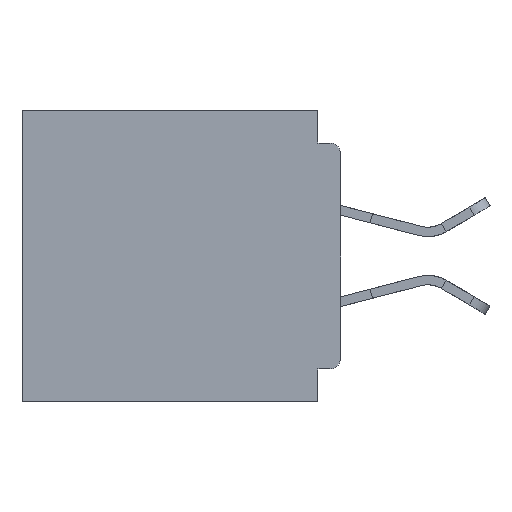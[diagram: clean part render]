
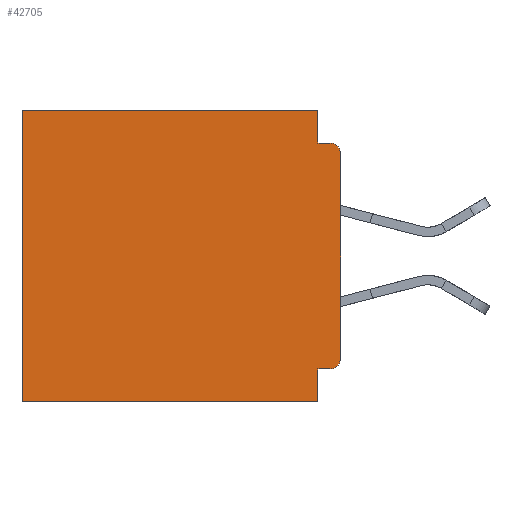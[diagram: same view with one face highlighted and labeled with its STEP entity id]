
A CAD part, left-side view. The second image highlights one B-rep face of the part: STEP entity #42705.
In plain terms, the highlighted planar face has unit normal (-1, 0, 0).
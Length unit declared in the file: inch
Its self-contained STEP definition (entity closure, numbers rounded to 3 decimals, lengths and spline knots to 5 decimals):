
#478 = ORIENTED_EDGE ( 'NONE', *, *, #38318, .T. ) ;
#631 = ORIENTED_EDGE ( 'NONE', *, *, #8554, .F. ) ;
#652 = ORIENTED_EDGE ( 'NONE', *, *, #33060, .F. ) ;
#1007 = ORIENTED_EDGE ( 'NONE', *, *, #11516, .F. ) ;
#1162 = DIRECTION ( 'NONE',  ( -1., 0., 0. ) ) ;
#1237 = DIRECTION ( 'NONE',  ( 0., 0., -1. ) ) ;
#1367 = LINE ( 'NONE', #6785, #37775 ) ;
#2070 = VERTEX_POINT ( 'NONE', #13846 ) ;
#2104 = LINE ( 'NONE', #34394, #11601 ) ;
#2105 = CARTESIAN_POINT ( 'NONE',  ( 0.3, 0.015, -0.045 ) ) ;
#2699 = VECTOR ( 'NONE', #28608, 39.37008 ) ;
#3477 = DIRECTION ( 'NONE',  ( 0., 0., -1. ) ) ;
#3554 = EDGE_CURVE ( 'NONE', #36889, #11849, #17380, .T. ) ;
#5534 = CARTESIAN_POINT ( 'NONE',  ( 0.3, 0., -0.4 ) ) ;
#6660 = VECTOR ( 'NONE', #39659, 39.37008 ) ;
#6785 = CARTESIAN_POINT ( 'NONE',  ( 0.3, 0.031, 0. ) ) ;
#8554 = EDGE_CURVE ( 'NONE', #10568, #42084, #30866, .T. ) ;
#8664 = ORIENTED_EDGE ( 'NONE', *, *, #3554, .T. ) ;
#9018 = ORIENTED_EDGE ( 'NONE', *, *, #45031, .F. ) ;
#9040 = LINE ( 'NONE', #41932, #25584 ) ;
#10282 = CIRCLE ( 'NONE', #40436, 0.015 ) ;
#10490 = CARTESIAN_POINT ( 'NONE',  ( 0.3, 0., -0.4 ) ) ;
#10568 = VERTEX_POINT ( 'NONE', #43877 ) ;
#11516 = EDGE_CURVE ( 'NONE', #36889, #31523, #1367, .T. ) ;
#11601 = VECTOR ( 'NONE', #37915, 39.37008 ) ;
#11849 = VERTEX_POINT ( 'NONE', #29709 ) ;
#12405 = VECTOR ( 'NONE', #40590, 39.37008 ) ;
#13846 = CARTESIAN_POINT ( 'NONE',  ( 0.3, 0.031, -0.4 ) ) ;
#17380 = LINE ( 'NONE', #35688, #25571 ) ;
#17696 = CARTESIAN_POINT ( 'NONE',  ( 0.3, 0., -0.34 ) ) ;
#17940 = ORIENTED_EDGE ( 'NONE', *, *, #24020, .F. ) ;
#18157 = VERTEX_POINT ( 'NONE', #43260 ) ;
#18740 = CARTESIAN_POINT ( 'NONE',  ( 0.3, 0.031, -0.4 ) ) ;
#19406 = DIRECTION ( 'NONE',  ( 0., -1., 0. ) ) ;
#20846 = ORIENTED_EDGE ( 'NONE', *, *, #22394, .T. ) ;
#21164 = PLANE ( 'NONE',  #26379 ) ;
#22394 = EDGE_CURVE ( 'NONE', #31267, #42084, #44136, .T. ) ;
#22407 = CARTESIAN_POINT ( 'NONE',  ( 0.3, 0.015, -0.06 ) ) ;
#22445 = EDGE_LOOP ( 'NONE', ( #631, #478, #9018, #1007, #8664, #24124, #652, #17940, #43235, #20846 ) ) ;
#22473 = DIRECTION ( 'NONE',  ( -1., 0., 0. ) ) ;
#22918 = CARTESIAN_POINT ( 'NONE',  ( 0.3, 0., -0.045 ) ) ;
#23870 = AXIS2_PLACEMENT_3D ( 'NONE', #43416, #22473, #1237 ) ;
#24020 = EDGE_CURVE ( 'NONE', #40606, #2070, #32587, .T. ) ;
#24117 = CARTESIAN_POINT ( 'NONE',  ( 0.3, 0.015, -0.355 ) ) ;
#24124 = ORIENTED_EDGE ( 'NONE', *, *, #38705, .T. ) ;
#24516 = DIRECTION ( 'NONE',  ( 0., 0., -1. ) ) ;
#24672 = DIRECTION ( 'NONE',  ( 1., 0., 0. ) ) ;
#24717 = FACE_OUTER_BOUND ( 'NONE', #22445, .T. ) ;
#24908 = EDGE_CURVE ( 'NONE', #31267, #40606, #2104, .T. ) ;
#25571 = VECTOR ( 'NONE', #35695, 39.37008 ) ;
#25584 = VECTOR ( 'NONE', #24516, 39.37008 ) ;
#25904 = DIRECTION ( 'NONE',  ( 0., 0., -1. ) ) ;
#26379 = AXIS2_PLACEMENT_3D ( 'NONE', #10490, #24672, #3477 ) ;
#28405 = VERTEX_POINT ( 'NONE', #2105 ) ;
#28608 = DIRECTION ( 'NONE',  ( 0., 0., -1. ) ) ;
#29709 = CARTESIAN_POINT ( 'NONE',  ( 0.3, 0.437, 0. ) ) ;
#30650 = CARTESIAN_POINT ( 'NONE',  ( 0.3, 0.031, -0.355 ) ) ;
#30866 = LINE ( 'NONE', #39024, #2699 ) ;
#31267 = VERTEX_POINT ( 'NONE', #24117 ) ;
#31523 = VERTEX_POINT ( 'NONE', #32037 ) ;
#32037 = CARTESIAN_POINT ( 'NONE',  ( 0.3, 0.031, -0.045 ) ) ;
#32587 = LINE ( 'NONE', #18740, #6660 ) ;
#33060 = EDGE_CURVE ( 'NONE', #2070, #18157, #39302, .T. ) ;
#34394 = CARTESIAN_POINT ( 'NONE',  ( 0.3, 0., -0.355 ) ) ;
#34937 = DIRECTION ( 'NONE',  ( 0., 0., -1. ) ) ;
#35688 = CARTESIAN_POINT ( 'NONE',  ( 0.3, 0., 0. ) ) ;
#35695 = DIRECTION ( 'NONE',  ( 0., 1., 0. ) ) ;
#36253 = VECTOR ( 'NONE', #19406, 39.37008 ) ;
#36889 = VERTEX_POINT ( 'NONE', #38479 ) ;
#37775 = VECTOR ( 'NONE', #34937, 39.37008 ) ;
#37915 = DIRECTION ( 'NONE',  ( 0., 1., 0. ) ) ;
#38318 = EDGE_CURVE ( 'NONE', #10568, #28405, #10282, .T. ) ;
#38479 = CARTESIAN_POINT ( 'NONE',  ( 0.3, 0.031, 0. ) ) ;
#38705 = EDGE_CURVE ( 'NONE', #11849, #18157, #9040, .T. ) ;
#39024 = CARTESIAN_POINT ( 'NONE',  ( 0.3, 0., -0.4 ) ) ;
#39302 = LINE ( 'NONE', #5534, #12405 ) ;
#39659 = DIRECTION ( 'NONE',  ( 0., 0., -1. ) ) ;
#40436 = AXIS2_PLACEMENT_3D ( 'NONE', #22407, #1162, #25904 ) ;
#40590 = DIRECTION ( 'NONE',  ( 0., 1., 0. ) ) ;
#40606 = VERTEX_POINT ( 'NONE', #30650 ) ;
#41932 = CARTESIAN_POINT ( 'NONE',  ( 0.3, 0.437, -0.4 ) ) ;
#42084 = VERTEX_POINT ( 'NONE', #17696 ) ;
#42705 = ADVANCED_FACE ( 'NONE', ( #24717 ), #21164, .F. ) ;
#43235 = ORIENTED_EDGE ( 'NONE', *, *, #24908, .F. ) ;
#43260 = CARTESIAN_POINT ( 'NONE',  ( 0.3, 0.437, -0.4 ) ) ;
#43416 = CARTESIAN_POINT ( 'NONE',  ( 0.3, 0.015, -0.34 ) ) ;
#43877 = CARTESIAN_POINT ( 'NONE',  ( 0.3, 0., -0.06 ) ) ;
#44136 = CIRCLE ( 'NONE', #23870, 0.015 ) ;
#45031 = EDGE_CURVE ( 'NONE', #31523, #28405, #45524, .T. ) ;
#45524 = LINE ( 'NONE', #22918, #36253 ) ;
